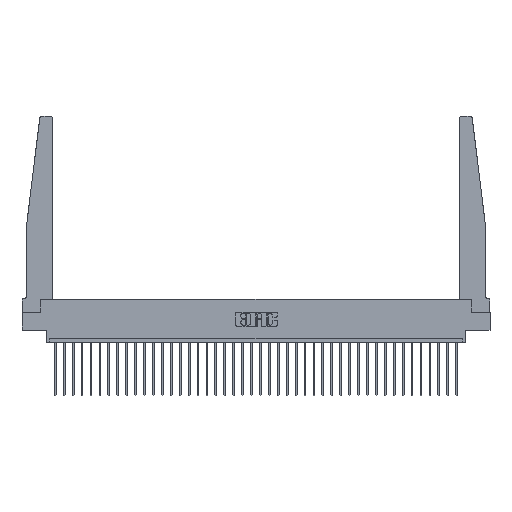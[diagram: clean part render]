
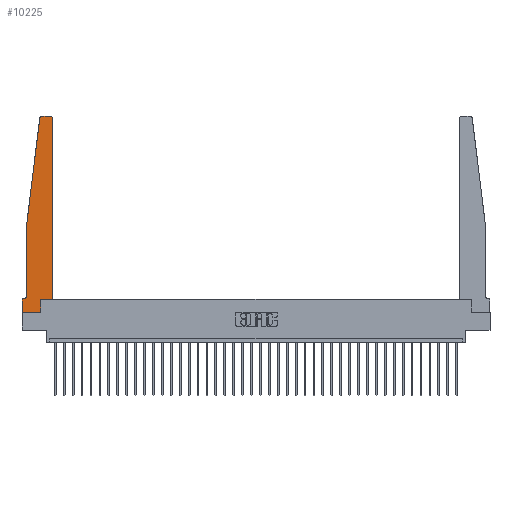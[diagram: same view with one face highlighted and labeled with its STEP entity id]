
A CAD part, top view. The second image highlights one B-rep face of the part: STEP entity #10225.
In plain terms, the highlighted planar face has unit normal (0, 0, 1).
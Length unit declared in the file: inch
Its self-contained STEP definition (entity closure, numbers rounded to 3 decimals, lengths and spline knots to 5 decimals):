
#866 = PLANE ( 'NONE',  #2168 ) ;
#966 = VERTEX_POINT ( 'NONE', #12955 ) ;
#1098 = ORIENTED_EDGE ( 'NONE', *, *, #27552, .T. ) ;
#1898 = CARTESIAN_POINT ( 'NONE',  ( 0., 0., 0.37 ) ) ;
#2168 = AXIS2_PLACEMENT_3D ( 'NONE', #21294, #18414, #6086 ) ;
#2503 = VERTEX_POINT ( 'NONE', #23947 ) ;
#2753 = ORIENTED_EDGE ( 'NONE', *, *, #2784, .T. ) ;
#2773 = ORIENTED_EDGE ( 'NONE', *, *, #23115, .T. ) ;
#2784 = EDGE_CURVE ( 'NONE', #28113, #966, #12916, .T. ) ;
#2933 = DIRECTION ( 'NONE',  ( -1., 0., 0. ) ) ;
#3872 = ORIENTED_EDGE ( 'NONE', *, *, #28014, .T. ) ;
#4031 = CARTESIAN_POINT ( 'NONE',  ( 0.065, 1.25, 0.37 ) ) ;
#4290 = EDGE_CURVE ( 'NONE', #31032, #14777, #32312, .T. ) ;
#4738 = VERTEX_POINT ( 'NONE', #18187 ) ;
#5070 = ORIENTED_EDGE ( 'NONE', *, *, #26235, .T. ) ;
#5972 = CARTESIAN_POINT ( 'NONE',  ( 0.015, 0.2375, 0.37 ) ) ;
#6086 = DIRECTION ( 'NONE',  ( 1., 0., 0. ) ) ;
#6133 = DIRECTION ( 'NONE',  ( 0., 0., -1. ) ) ;
#6206 = VERTEX_POINT ( 'NONE', #27962 ) ;
#6364 = DIRECTION ( 'NONE',  ( 0., 1., 0. ) ) ;
#6817 = VECTOR ( 'NONE', #11127, 39.37008 ) ;
#7275 = VERTEX_POINT ( 'NONE', #23984 ) ;
#7631 = CARTESIAN_POINT ( 'NONE',  ( 0.24675, 2.72367, 0.37 ) ) ;
#7680 = VERTEX_POINT ( 'NONE', #33226 ) ;
#7947 = FACE_OUTER_BOUND ( 'NONE', #17427, .T. ) ;
#8093 = DIRECTION ( 'NONE',  ( 0., 0., 1. ) ) ;
#9107 = LINE ( 'NONE', #4031, #6817 ) ;
#9296 = CARTESIAN_POINT ( 'NONE',  ( 0.065, 1.25, 0.37 ) ) ;
#9367 = DIRECTION ( 'NONE',  ( 1., 0., 0. ) ) ;
#9718 = CARTESIAN_POINT ( 'NONE',  ( 0.27653, 2.72, 0.37 ) ) ;
#9982 = CARTESIAN_POINT ( 'NONE',  ( 0.25, 2.75, 0.37 ) ) ;
#10043 = DIRECTION ( 'NONE',  ( 0., 0., 1. ) ) ;
#10225 = ADVANCED_FACE ( 'NONE', ( #7947 ), #866, .T. ) ;
#10959 = CARTESIAN_POINT ( 'NONE',  ( 0., 0.1875, 0.37 ) ) ;
#11127 = DIRECTION ( 'NONE',  ( 0., -1., 0. ) ) ;
#11352 = EDGE_CURVE ( 'NONE', #18269, #28113, #30921, .T. ) ;
#11424 = LINE ( 'NONE', #14113, #22617 ) ;
#11698 = ORIENTED_EDGE ( 'NONE', *, *, #33364, .T. ) ;
#11709 = ORIENTED_EDGE ( 'NONE', *, *, #17896, .T. ) ;
#12526 = LINE ( 'NONE', #22852, #25006 ) ;
#12916 = LINE ( 'NONE', #33037, #29908 ) ;
#12955 = CARTESIAN_POINT ( 'NONE',  ( 0.2605, 0.18, 0.37 ) ) ;
#14113 = CARTESIAN_POINT ( 'NONE',  ( 0.425, 0.18, 0.37 ) ) ;
#14777 = VERTEX_POINT ( 'NONE', #32732 ) ;
#14968 = VECTOR ( 'NONE', #16474, 39.37008 ) ;
#15732 = DIRECTION ( 'NONE',  ( 1., 0., 0. ) ) ;
#15888 = ORIENTED_EDGE ( 'NONE', *, *, #11352, .T. ) ;
#15895 = CARTESIAN_POINT ( 'NONE',  ( 0., 0., 0.37 ) ) ;
#16474 = DIRECTION ( 'NONE',  ( 0., -1., 0. ) ) ;
#17291 = VECTOR ( 'NONE', #9367, 39.37008 ) ;
#17427 = EDGE_LOOP ( 'NONE', ( #25846, #28254, #11698, #2773, #1098, #11709, #5070, #15888, #2753, #32079, #3872, #25713 ) ) ;
#17896 = EDGE_CURVE ( 'NONE', #2503, #22871, #12526, .T. ) ;
#18187 = CARTESIAN_POINT ( 'NONE',  ( 0.065, 0.2375, 0.37 ) ) ;
#18269 = VERTEX_POINT ( 'NONE', #1898 ) ;
#18414 = DIRECTION ( 'NONE',  ( 0., 0., 1. ) ) ;
#19014 = LINE ( 'NONE', #29316, #14968 ) ;
#20212 = DIRECTION ( 'NONE',  ( 0., 1., 0. ) ) ;
#20283 = DIRECTION ( 'NONE',  ( -1., 0., 0. ) ) ;
#21294 = CARTESIAN_POINT ( 'NONE',  ( 0., 0.1875, 0.37 ) ) ;
#21506 = CARTESIAN_POINT ( 'NONE',  ( 0.425, 2.72, 0.37 ) ) ;
#22354 = VERTEX_POINT ( 'NONE', #7631 ) ;
#22617 = VECTOR ( 'NONE', #6364, 39.37008 ) ;
#22852 = CARTESIAN_POINT ( 'NONE',  ( 0.065, 0.1875, 0.37 ) ) ;
#22871 = VERTEX_POINT ( 'NONE', #10959 ) ;
#23115 = EDGE_CURVE ( 'NONE', #7275, #4738, #9107, .T. ) ;
#23416 = EDGE_CURVE ( 'NONE', #6206, #22354, #30527, .T. ) ;
#23947 = CARTESIAN_POINT ( 'NONE',  ( 0.015, 0.1875, 0.37 ) ) ;
#23969 = DIRECTION ( 'NONE',  ( 1., 0., 0. ) ) ;
#23984 = CARTESIAN_POINT ( 'NONE',  ( 0.065, 1.25, 0.37 ) ) ;
#24565 = LINE ( 'NONE', #27432, #17291 ) ;
#24995 = LINE ( 'NONE', #9296, #25616 ) ;
#25006 = VECTOR ( 'NONE', #33142, 39.37008 ) ;
#25307 = AXIS2_PLACEMENT_3D ( 'NONE', #25988, #8093, #23969 ) ;
#25616 = VECTOR ( 'NONE', #27361, 39.37008 ) ;
#25713 = ORIENTED_EDGE ( 'NONE', *, *, #4290, .T. ) ;
#25810 = CIRCLE ( 'NONE', #31735, 0.05 ) ;
#25846 = ORIENTED_EDGE ( 'NONE', *, *, #32013, .T. ) ;
#25988 = CARTESIAN_POINT ( 'NONE',  ( 0.395, 2.72, 0.37 ) ) ;
#26235 = EDGE_CURVE ( 'NONE', #22871, #18269, #19014, .T. ) ;
#27361 = DIRECTION ( 'NONE',  ( -0.122, -0.992, 0. ) ) ;
#27432 = CARTESIAN_POINT ( 'NONE',  ( 0.425, 0.18, 0.37 ) ) ;
#27552 = EDGE_CURVE ( 'NONE', #4738, #2503, #25810, .T. ) ;
#27962 = CARTESIAN_POINT ( 'NONE',  ( 0.27653, 2.75, 0.37 ) ) ;
#28014 = EDGE_CURVE ( 'NONE', #7680, #31032, #11424, .T. ) ;
#28113 = VERTEX_POINT ( 'NONE', #29989 ) ;
#28254 = ORIENTED_EDGE ( 'NONE', *, *, #23416, .T. ) ;
#29316 = CARTESIAN_POINT ( 'NONE',  ( 0., 0., 0.37 ) ) ;
#29608 = EDGE_CURVE ( 'NONE', #966, #7680, #24565, .T. ) ;
#29908 = VECTOR ( 'NONE', #20212, 39.37008 ) ;
#29989 = CARTESIAN_POINT ( 'NONE',  ( 0.2605, 0., 0.37 ) ) ;
#30017 = AXIS2_PLACEMENT_3D ( 'NONE', #9718, #10043, #30306 ) ;
#30306 = DIRECTION ( 'NONE',  ( 1., 0., 0. ) ) ;
#30527 = CIRCLE ( 'NONE', #30017, 0.03 ) ;
#30921 = LINE ( 'NONE', #15895, #31766 ) ;
#31032 = VERTEX_POINT ( 'NONE', #21506 ) ;
#31735 = AXIS2_PLACEMENT_3D ( 'NONE', #5972, #6133, #2933 ) ;
#31766 = VECTOR ( 'NONE', #15732, 39.37008 ) ;
#32013 = EDGE_CURVE ( 'NONE', #14777, #6206, #33110, .T. ) ;
#32079 = ORIENTED_EDGE ( 'NONE', *, *, #29608, .T. ) ;
#32312 = CIRCLE ( 'NONE', #25307, 0.03 ) ;
#32390 = VECTOR ( 'NONE', #20283, 39.37008 ) ;
#32732 = CARTESIAN_POINT ( 'NONE',  ( 0.395, 2.75, 0.37 ) ) ;
#33037 = CARTESIAN_POINT ( 'NONE',  ( 0.2605, 0.18, 0.37 ) ) ;
#33110 = LINE ( 'NONE', #9982, #32390 ) ;
#33142 = DIRECTION ( 'NONE',  ( -1., 0., 0. ) ) ;
#33226 = CARTESIAN_POINT ( 'NONE',  ( 0.425, 0.18, 0.37 ) ) ;
#33364 = EDGE_CURVE ( 'NONE', #22354, #7275, #24995, .T. ) ;
